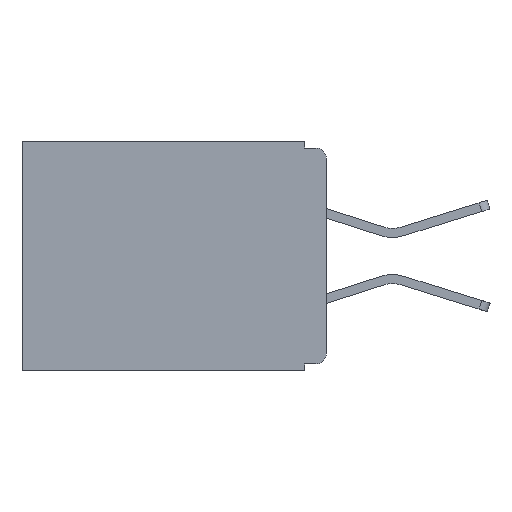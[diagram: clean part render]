
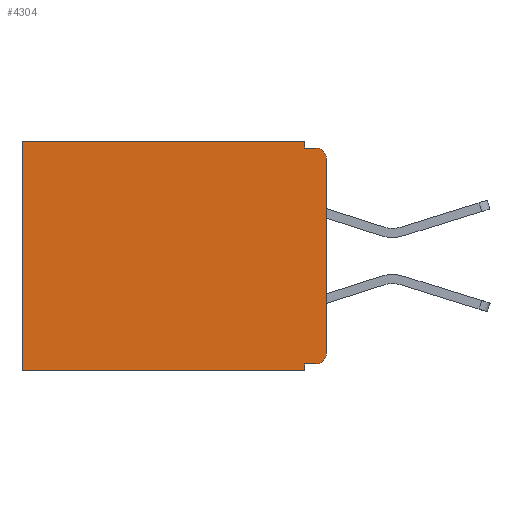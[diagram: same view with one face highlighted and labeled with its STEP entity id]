
A CAD part, left-side view. The second image highlights one B-rep face of the part: STEP entity #4304.
In plain terms, the highlighted planar face has unit normal (-1, 0, 0).
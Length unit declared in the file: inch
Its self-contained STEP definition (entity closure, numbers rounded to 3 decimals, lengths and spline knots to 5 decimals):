
#21 = DIRECTION ( 'NONE',  ( 0., 0., -1. ) ) ;
#33 = VECTOR ( 'NONE', #7167, 39.37008 ) ;
#138 = FACE_OUTER_BOUND ( 'NONE', #3347, .T. ) ;
#203 = EDGE_CURVE ( 'NONE', #5490, #2754, #8386, .T. ) ;
#277 = VECTOR ( 'NONE', #2852, 39.37008 ) ;
#771 = EDGE_CURVE ( 'NONE', #3083, #2187, #7509, .T. ) ;
#1014 = VECTOR ( 'NONE', #2652, 39.37008 ) ;
#1261 = LINE ( 'NONE', #7395, #33 ) ;
#1398 = VECTOR ( 'NONE', #6624, 39.37008 ) ;
#1762 = ORIENTED_EDGE ( 'NONE', *, *, #2811, .F. ) ;
#1799 = CARTESIAN_POINT ( 'NONE',  ( 0.3, 0., -0.305 ) ) ;
#1806 = CARTESIAN_POINT ( 'NONE',  ( 0.3, 0.437, -0.33 ) ) ;
#1908 = VECTOR ( 'NONE', #4011, 39.37008 ) ;
#2038 = VERTEX_POINT ( 'NONE', #2845 ) ;
#2182 = EDGE_CURVE ( 'NONE', #2187, #9732, #1261, .T. ) ;
#2187 = VERTEX_POINT ( 'NONE', #7347 ) ;
#2219 = CARTESIAN_POINT ( 'NONE',  ( 0.3, 0.015, -0.32 ) ) ;
#2398 = CARTESIAN_POINT ( 'NONE',  ( 0.3, 0., 0. ) ) ;
#2544 = VECTOR ( 'NONE', #8144, 39.37008 ) ;
#2577 = ORIENTED_EDGE ( 'NONE', *, *, #9257, .F. ) ;
#2620 = ORIENTED_EDGE ( 'NONE', *, *, #10469, .T. ) ;
#2652 = DIRECTION ( 'NONE',  ( 0., 1., 0. ) ) ;
#2734 = CARTESIAN_POINT ( 'NONE',  ( 0.3, 0.437, -0.33 ) ) ;
#2754 = VERTEX_POINT ( 'NONE', #6015 ) ;
#2811 = EDGE_CURVE ( 'NONE', #9732, #7018, #10858, .T. ) ;
#2845 = CARTESIAN_POINT ( 'NONE',  ( 0.3, 0.015, -0.01 ) ) ;
#2848 = ORIENTED_EDGE ( 'NONE', *, *, #203, .T. ) ;
#2852 = DIRECTION ( 'NONE',  ( 0., 0., -1. ) ) ;
#2970 = VECTOR ( 'NONE', #5793, 39.37008 ) ;
#3083 = VERTEX_POINT ( 'NONE', #2219 ) ;
#3159 = ORIENTED_EDGE ( 'NONE', *, *, #2182, .F. ) ;
#3334 = CARTESIAN_POINT ( 'NONE',  ( 0.3, 0., -0.33 ) ) ;
#3347 = EDGE_LOOP ( 'NONE', ( #9655, #3457, #2577, #4909, #2848, #6318, #1762, #3159, #11572, #2620 ) ) ;
#3457 = ORIENTED_EDGE ( 'NONE', *, *, #9615, .T. ) ;
#3514 = VERTEX_POINT ( 'NONE', #1799 ) ;
#3570 = CIRCLE ( 'NONE', #7366, 0.015 ) ;
#3574 = CARTESIAN_POINT ( 'NONE',  ( 0.3, 0.031, -0.33 ) ) ;
#4011 = DIRECTION ( 'NONE',  ( 0., 0., -1. ) ) ;
#4046 = CARTESIAN_POINT ( 'NONE',  ( 0.3, 0., -0.32 ) ) ;
#4281 = DIRECTION ( 'NONE',  ( -1., 0., 0. ) ) ;
#4304 = ADVANCED_FACE ( 'NONE', ( #138 ), #11860, .F. ) ;
#4401 = AXIS2_PLACEMENT_3D ( 'NONE', #9690, #4281, #10601 ) ;
#4504 = VERTEX_POINT ( 'NONE', #9941 ) ;
#4737 = LINE ( 'NONE', #8499, #2544 ) ;
#4909 = ORIENTED_EDGE ( 'NONE', *, *, #5027, .F. ) ;
#5027 = EDGE_CURVE ( 'NONE', #5490, #4504, #4737, .T. ) ;
#5490 = VERTEX_POINT ( 'NONE', #7502 ) ;
#5640 = CARTESIAN_POINT ( 'NONE',  ( 0.3, 0., -0.01 ) ) ;
#5698 = DIRECTION ( 'NONE',  ( -1., 0., 0. ) ) ;
#5793 = DIRECTION ( 'NONE',  ( 0., 1., 0. ) ) ;
#6015 = CARTESIAN_POINT ( 'NONE',  ( 0.3, 0.437, 0. ) ) ;
#6265 = EDGE_CURVE ( 'NONE', #11593, #3514, #11318, .T. ) ;
#6318 = ORIENTED_EDGE ( 'NONE', *, *, #8507, .T. ) ;
#6624 = DIRECTION ( 'NONE',  ( 0., 1., 0. ) ) ;
#6650 = CARTESIAN_POINT ( 'NONE',  ( 0.3, 0., -0.33 ) ) ;
#7018 = VERTEX_POINT ( 'NONE', #1806 ) ;
#7167 = DIRECTION ( 'NONE',  ( 0., 0., -1. ) ) ;
#7347 = CARTESIAN_POINT ( 'NONE',  ( 0.3, 0.031, -0.32 ) ) ;
#7366 = AXIS2_PLACEMENT_3D ( 'NONE', #11072, #5698, #21 ) ;
#7395 = CARTESIAN_POINT ( 'NONE',  ( 0.3, 0.031, -0.33 ) ) ;
#7414 = LINE ( 'NONE', #2734, #277 ) ;
#7502 = CARTESIAN_POINT ( 'NONE',  ( 0.3, 0.031, 0. ) ) ;
#7509 = LINE ( 'NONE', #4046, #2970 ) ;
#7528 = CIRCLE ( 'NONE', #4401, 0.015 ) ;
#7895 = DIRECTION ( 'NONE',  ( 0., 0., -1. ) ) ;
#8144 = DIRECTION ( 'NONE',  ( 0., 0., -1. ) ) ;
#8352 = DIRECTION ( 'NONE',  ( 0., -1., 0. ) ) ;
#8386 = LINE ( 'NONE', #2398, #1014 ) ;
#8499 = CARTESIAN_POINT ( 'NONE',  ( 0.3, 0.031, 0. ) ) ;
#8507 = EDGE_CURVE ( 'NONE', #2754, #7018, #7414, .T. ) ;
#8537 = VECTOR ( 'NONE', #8352, 39.37008 ) ;
#9051 = CARTESIAN_POINT ( 'NONE',  ( 0.3, 0., -0.025 ) ) ;
#9257 = EDGE_CURVE ( 'NONE', #4504, #2038, #10934, .T. ) ;
#9446 = DIRECTION ( 'NONE',  ( 1., 0., 0. ) ) ;
#9615 = EDGE_CURVE ( 'NONE', #11593, #2038, #7528, .T. ) ;
#9655 = ORIENTED_EDGE ( 'NONE', *, *, #6265, .F. ) ;
#9690 = CARTESIAN_POINT ( 'NONE',  ( 0.3, 0.015, -0.025 ) ) ;
#9732 = VERTEX_POINT ( 'NONE', #3574 ) ;
#9941 = CARTESIAN_POINT ( 'NONE',  ( 0.3, 0.031, -0.01 ) ) ;
#9998 = AXIS2_PLACEMENT_3D ( 'NONE', #3334, #9446, #7895 ) ;
#10373 = CARTESIAN_POINT ( 'NONE',  ( 0.3, 0., -0.33 ) ) ;
#10469 = EDGE_CURVE ( 'NONE', #3083, #3514, #3570, .T. ) ;
#10601 = DIRECTION ( 'NONE',  ( 0., 0., -1. ) ) ;
#10858 = LINE ( 'NONE', #6650, #1398 ) ;
#10934 = LINE ( 'NONE', #5640, #8537 ) ;
#11072 = CARTESIAN_POINT ( 'NONE',  ( 0.3, 0.015, -0.305 ) ) ;
#11318 = LINE ( 'NONE', #10373, #1908 ) ;
#11572 = ORIENTED_EDGE ( 'NONE', *, *, #771, .F. ) ;
#11593 = VERTEX_POINT ( 'NONE', #9051 ) ;
#11860 = PLANE ( 'NONE',  #9998 ) ;
